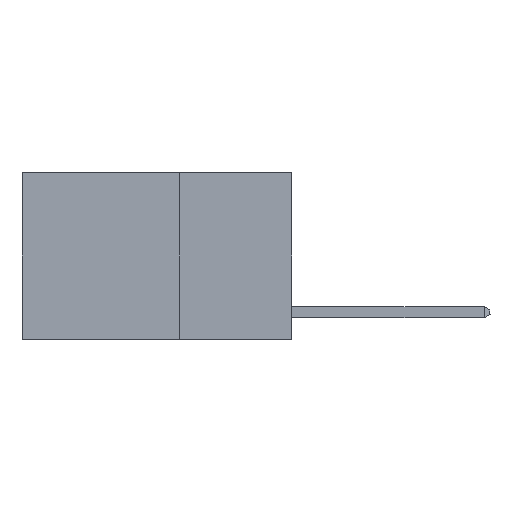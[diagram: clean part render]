
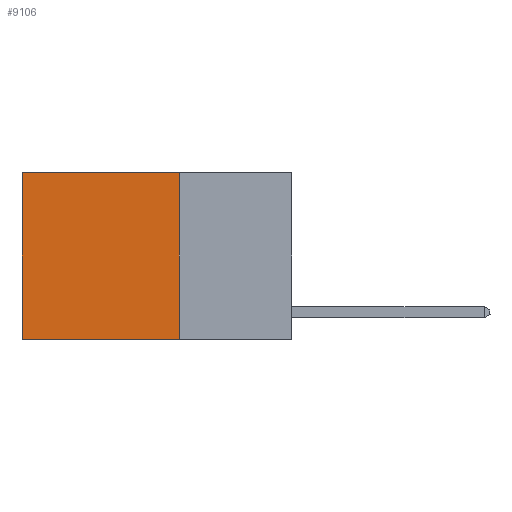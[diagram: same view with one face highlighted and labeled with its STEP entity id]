
A CAD part, left-side view. The second image highlights one B-rep face of the part: STEP entity #9106.
In plain terms, the highlighted planar face has unit normal (-1, 0, 0).
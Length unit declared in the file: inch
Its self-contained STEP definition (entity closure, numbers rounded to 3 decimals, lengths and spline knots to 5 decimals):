
#514 = EDGE_CURVE ( 'NONE', #4003, #10710, #5336, .T. ) ;
#1694 = DIRECTION ( 'NONE',  ( 0., 1., 0. ) ) ;
#1723 = LINE ( 'NONE', #2865, #5939 ) ;
#1931 = DIRECTION ( 'NONE',  ( 0., 1., 0. ) ) ;
#2275 = DIRECTION ( 'NONE',  ( 0., 0., -1. ) ) ;
#2550 = ORIENTED_EDGE ( 'NONE', *, *, #8921, .T. ) ;
#2743 = AXIS2_PLACEMENT_3D ( 'NONE', #2903, #3938, #8238 ) ;
#2804 = ORIENTED_EDGE ( 'NONE', *, *, #3705, .T. ) ;
#2865 = CARTESIAN_POINT ( 'NONE',  ( 0.2625, 0.25, -0.37 ) ) ;
#2903 = CARTESIAN_POINT ( 'NONE',  ( 0.2625, 0.25, 0. ) ) ;
#3705 = EDGE_CURVE ( 'NONE', #4688, #13206, #7464, .T. ) ;
#3938 = DIRECTION ( 'NONE',  ( 1., 0., 0. ) ) ;
#4003 = VERTEX_POINT ( 'NONE', #11738 ) ;
#4285 = CARTESIAN_POINT ( 'NONE',  ( 0.2625, 0.25, -0.37 ) ) ;
#4358 = CARTESIAN_POINT ( 'NONE',  ( 0.2625, 0.6, -0.37 ) ) ;
#4688 = VERTEX_POINT ( 'NONE', #6045 ) ;
#4753 = CARTESIAN_POINT ( 'NONE',  ( 0.2625, 0.25, 0. ) ) ;
#5336 = LINE ( 'NONE', #9456, #12262 ) ;
#5939 = VECTOR ( 'NONE', #1931, 39.37008 ) ;
#6045 = CARTESIAN_POINT ( 'NONE',  ( 0.2625, 0.6, 0. ) ) ;
#6261 = FACE_OUTER_BOUND ( 'NONE', #8381, .T. ) ;
#7112 = VECTOR ( 'NONE', #2275, 39.37008 ) ;
#7464 = LINE ( 'NONE', #11640, #7112 ) ;
#7724 = ORIENTED_EDGE ( 'NONE', *, *, #8180, .F. ) ;
#7877 = LINE ( 'NONE', #4753, #12796 ) ;
#8180 = EDGE_CURVE ( 'NONE', #10710, #13206, #1723, .T. ) ;
#8238 = DIRECTION ( 'NONE',  ( 0., 0., -1. ) ) ;
#8371 = PLANE ( 'NONE',  #2743 ) ;
#8381 = EDGE_LOOP ( 'NONE', ( #2804, #7724, #12117, #2550 ) ) ;
#8921 = EDGE_CURVE ( 'NONE', #4003, #4688, #7877, .T. ) ;
#9106 = ADVANCED_FACE ( 'NONE', ( #6261 ), #8371, .F. ) ;
#9456 = CARTESIAN_POINT ( 'NONE',  ( 0.2625, 0.25, 0. ) ) ;
#10710 = VERTEX_POINT ( 'NONE', #4285 ) ;
#11427 = DIRECTION ( 'NONE',  ( 0., 0., -1. ) ) ;
#11640 = CARTESIAN_POINT ( 'NONE',  ( 0.2625, 0.6, 0. ) ) ;
#11738 = CARTESIAN_POINT ( 'NONE',  ( 0.2625, 0.25, 0. ) ) ;
#12117 = ORIENTED_EDGE ( 'NONE', *, *, #514, .F. ) ;
#12262 = VECTOR ( 'NONE', #11427, 39.37008 ) ;
#12796 = VECTOR ( 'NONE', #1694, 39.37008 ) ;
#13206 = VERTEX_POINT ( 'NONE', #4358 ) ;
